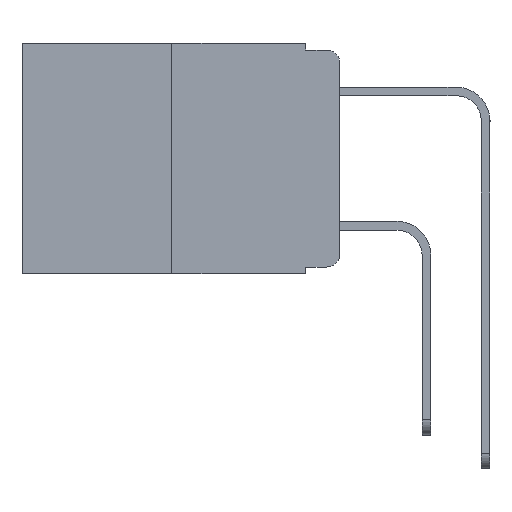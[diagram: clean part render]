
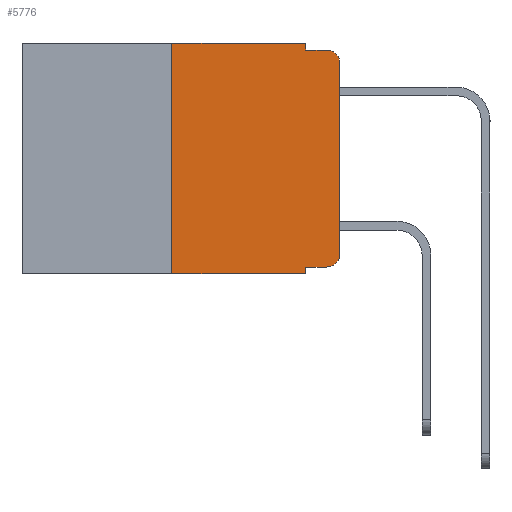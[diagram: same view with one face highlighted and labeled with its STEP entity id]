
A CAD part, left-side view. The second image highlights one B-rep face of the part: STEP entity #5776.
In plain terms, the highlighted planar face has unit normal (-1, 0, 0).
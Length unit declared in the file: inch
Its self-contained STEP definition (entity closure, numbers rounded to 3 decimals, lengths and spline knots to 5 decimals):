
#16 = DIRECTION ( 'NONE',  ( 0., 0., -1. ) ) ;
#53 = VERTEX_POINT ( 'NONE', #5259 ) ;
#278 = DIRECTION ( 'NONE',  ( 0., -1., 0. ) ) ;
#298 = CARTESIAN_POINT ( 'NONE',  ( 0., 0.473, 0. ) ) ;
#305 = VECTOR ( 'NONE', #17555, 39.37008 ) ;
#450 = CARTESIAN_POINT ( 'NONE',  ( 0., 0.02, -0.01 ) ) ;
#801 = ORIENTED_EDGE ( 'NONE', *, *, #17601, .T. ) ;
#947 = VERTEX_POINT ( 'NONE', #16538 ) ;
#1562 = VERTEX_POINT ( 'NONE', #10600 ) ;
#1675 = LINE ( 'NONE', #8579, #5517 ) ;
#1696 = VERTEX_POINT ( 'NONE', #2315 ) ;
#1782 = DIRECTION ( 'NONE',  ( 1., 0., 0. ) ) ;
#2226 = FACE_OUTER_BOUND ( 'NONE', #14456, .T. ) ;
#2315 = CARTESIAN_POINT ( 'NONE',  ( 0., 0.051, -0.333 ) ) ;
#2563 = DIRECTION ( 'NONE',  ( -1., 0., 0. ) ) ;
#2614 = VERTEX_POINT ( 'NONE', #5190 ) ;
#2622 = CIRCLE ( 'NONE', #13780, 0.02 ) ;
#2969 = VERTEX_POINT ( 'NONE', #16376 ) ;
#3396 = VERTEX_POINT ( 'NONE', #12177 ) ;
#3523 = VECTOR ( 'NONE', #278, 39.37008 ) ;
#4212 = LINE ( 'NONE', #5530, #305 ) ;
#4530 = VECTOR ( 'NONE', #12094, 39.37008 ) ;
#4942 = CARTESIAN_POINT ( 'NONE',  ( 0., 0.25, -0.343 ) ) ;
#5188 = VERTEX_POINT ( 'NONE', #11155 ) ;
#5190 = CARTESIAN_POINT ( 'NONE',  ( 0., 0., -0.03 ) ) ;
#5222 = DIRECTION ( 'NONE',  ( 0., -1., 0. ) ) ;
#5243 = DIRECTION ( 'NONE',  ( 0., 0., 1. ) ) ;
#5259 = CARTESIAN_POINT ( 'NONE',  ( 0., 0.051, 0. ) ) ;
#5285 = LINE ( 'NONE', #13401, #12085 ) ;
#5339 = VERTEX_POINT ( 'NONE', #4942 ) ;
#5517 = VECTOR ( 'NONE', #16, 39.37008 ) ;
#5530 = CARTESIAN_POINT ( 'NONE',  ( 0., 0.473, 0. ) ) ;
#5776 = ADVANCED_FACE ( 'NONE', ( #2226 ), #8820, .F. ) ;
#5892 = VECTOR ( 'NONE', #15769, 39.37008 ) ;
#6681 = ORIENTED_EDGE ( 'NONE', *, *, #11904, .T. ) ;
#6981 = VECTOR ( 'NONE', #5222, 39.37008 ) ;
#7136 = VERTEX_POINT ( 'NONE', #450 ) ;
#7203 = EDGE_CURVE ( 'NONE', #3396, #2969, #2622, .T. ) ;
#7527 = ORIENTED_EDGE ( 'NONE', *, *, #11157, .F. ) ;
#7764 = CARTESIAN_POINT ( 'NONE',  ( 0., 0.02, -0.313 ) ) ;
#8117 = EDGE_CURVE ( 'NONE', #1696, #5188, #1675, .T. ) ;
#8219 = LINE ( 'NONE', #17406, #4530 ) ;
#8413 = CIRCLE ( 'NONE', #9272, 0.02 ) ;
#8579 = CARTESIAN_POINT ( 'NONE',  ( 0., 0.051, 0. ) ) ;
#8793 = EDGE_CURVE ( 'NONE', #2969, #2614, #5285, .T. ) ;
#8811 = ORIENTED_EDGE ( 'NONE', *, *, #8117, .F. ) ;
#8820 = PLANE ( 'NONE',  #17156 ) ;
#9115 = DIRECTION ( 'NONE',  ( 0., 0., -1. ) ) ;
#9272 = AXIS2_PLACEMENT_3D ( 'NONE', #10894, #2563, #12250 ) ;
#9505 = LINE ( 'NONE', #13085, #5892 ) ;
#10164 = CARTESIAN_POINT ( 'NONE',  ( 0., 0.051, -0.01 ) ) ;
#10300 = VECTOR ( 'NONE', #16155, 39.37008 ) ;
#10600 = CARTESIAN_POINT ( 'NONE',  ( 0., 0.25, 0. ) ) ;
#10705 = ORIENTED_EDGE ( 'NONE', *, *, #16322, .F. ) ;
#10894 = CARTESIAN_POINT ( 'NONE',  ( 0., 0.02, -0.03 ) ) ;
#11113 = ORIENTED_EDGE ( 'NONE', *, *, #13893, .F. ) ;
#11155 = CARTESIAN_POINT ( 'NONE',  ( 0., 0.051, -0.343 ) ) ;
#11157 = EDGE_CURVE ( 'NONE', #53, #947, #8219, .T. ) ;
#11518 = DIRECTION ( 'NONE',  ( 0., 0., -1. ) ) ;
#11538 = ORIENTED_EDGE ( 'NONE', *, *, #17449, .F. ) ;
#11904 = EDGE_CURVE ( 'NONE', #2614, #7136, #8413, .T. ) ;
#12085 = VECTOR ( 'NONE', #5243, 39.37008 ) ;
#12094 = DIRECTION ( 'NONE',  ( 0., 0., -1. ) ) ;
#12177 = CARTESIAN_POINT ( 'NONE',  ( 0., 0.02, -0.333 ) ) ;
#12250 = DIRECTION ( 'NONE',  ( 0., 0., -1. ) ) ;
#12514 = EDGE_CURVE ( 'NONE', #5339, #5188, #13908, .T. ) ;
#13085 = CARTESIAN_POINT ( 'NONE',  ( 0., 0.25, 0. ) ) ;
#13187 = LINE ( 'NONE', #10164, #3523 ) ;
#13401 = CARTESIAN_POINT ( 'NONE',  ( 0., 0., 0. ) ) ;
#13780 = AXIS2_PLACEMENT_3D ( 'NONE', #7764, #17118, #9115 ) ;
#13893 = EDGE_CURVE ( 'NONE', #1562, #53, #4212, .T. ) ;
#13908 = LINE ( 'NONE', #14866, #10300 ) ;
#14456 = EDGE_LOOP ( 'NONE', ( #16560, #6681, #10705, #7527, #11113, #11538, #15154, #8811, #801, #15961 ) ) ;
#14866 = CARTESIAN_POINT ( 'NONE',  ( 0., 0.473, -0.343 ) ) ;
#15154 = ORIENTED_EDGE ( 'NONE', *, *, #12514, .T. ) ;
#15769 = DIRECTION ( 'NONE',  ( 0., 0., 1. ) ) ;
#15961 = ORIENTED_EDGE ( 'NONE', *, *, #7203, .T. ) ;
#16155 = DIRECTION ( 'NONE',  ( 0., -1., 0. ) ) ;
#16322 = EDGE_CURVE ( 'NONE', #947, #7136, #13187, .T. ) ;
#16376 = CARTESIAN_POINT ( 'NONE',  ( 0., 0., -0.313 ) ) ;
#16538 = CARTESIAN_POINT ( 'NONE',  ( 0., 0.051, -0.01 ) ) ;
#16560 = ORIENTED_EDGE ( 'NONE', *, *, #8793, .T. ) ;
#17118 = DIRECTION ( 'NONE',  ( -1., 0., 0. ) ) ;
#17156 = AXIS2_PLACEMENT_3D ( 'NONE', #298, #1782, #11518 ) ;
#17324 = CARTESIAN_POINT ( 'NONE',  ( 0., 0.051, -0.333 ) ) ;
#17406 = CARTESIAN_POINT ( 'NONE',  ( 0., 0.051, 0. ) ) ;
#17449 = EDGE_CURVE ( 'NONE', #5339, #1562, #9505, .T. ) ;
#17555 = DIRECTION ( 'NONE',  ( 0., -1., 0. ) ) ;
#17601 = EDGE_CURVE ( 'NONE', #1696, #3396, #17617, .T. ) ;
#17617 = LINE ( 'NONE', #17324, #6981 ) ;
